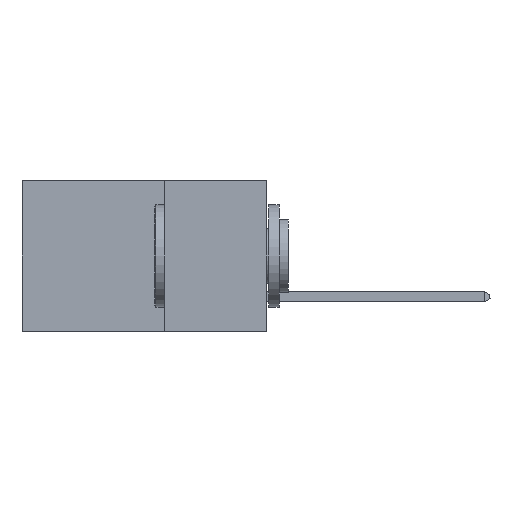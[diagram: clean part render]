
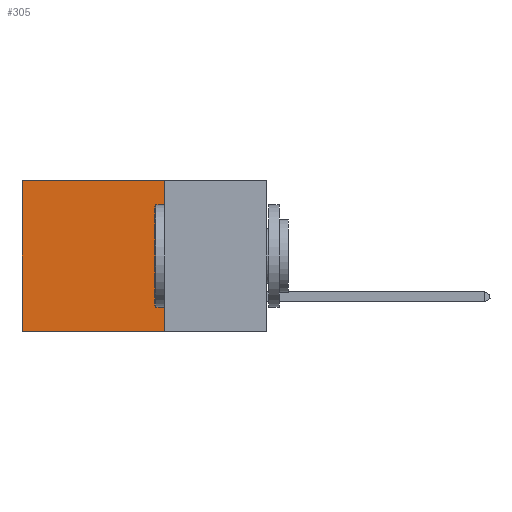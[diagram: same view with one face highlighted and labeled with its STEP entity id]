
A CAD part, left-side view. The second image highlights one B-rep face of the part: STEP entity #305.
In plain terms, the highlighted planar face has unit normal (-1, 0, 0).
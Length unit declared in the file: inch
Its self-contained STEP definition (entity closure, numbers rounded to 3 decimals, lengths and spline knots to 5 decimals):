
#305 = ADVANCED_FACE ( 'NONE', ( #17770 ), #11536, .F. ) ;
#1922 = ORIENTED_EDGE ( 'NONE', *, *, #16157, .F. ) ;
#2717 = EDGE_LOOP ( 'NONE', ( #24050, #1922, #35778, #18576 ) ) ;
#6690 = VERTEX_POINT ( 'NONE', #21975 ) ;
#7253 = LINE ( 'NONE', #20893, #22119 ) ;
#8516 = CARTESIAN_POINT ( 'NONE',  ( 0.2875, 0.25, 0. ) ) ;
#11536 = PLANE ( 'NONE',  #38023 ) ;
#11896 = CARTESIAN_POINT ( 'NONE',  ( 0.2875, 0.25, 0. ) ) ;
#12850 = LINE ( 'NONE', #30334, #37197 ) ;
#16157 = EDGE_CURVE ( 'NONE', #17183, #26474, #7253, .T. ) ;
#17183 = VERTEX_POINT ( 'NONE', #22636 ) ;
#17770 = FACE_OUTER_BOUND ( 'NONE', #2717, .T. ) ;
#18576 = ORIENTED_EDGE ( 'NONE', *, *, #26030, .T. ) ;
#19178 = LINE ( 'NONE', #8516, #35517 ) ;
#20381 = DIRECTION ( 'NONE',  ( 0., 0., -1. ) ) ;
#20893 = CARTESIAN_POINT ( 'NONE',  ( 0.2875, 0.25, -0.37 ) ) ;
#20948 = CARTESIAN_POINT ( 'NONE',  ( 0.2875, 0.25, 0. ) ) ;
#21975 = CARTESIAN_POINT ( 'NONE',  ( 0.2875, 0.6, 0. ) ) ;
#22119 = VECTOR ( 'NONE', #27307, 39.37008 ) ;
#22636 = CARTESIAN_POINT ( 'NONE',  ( 0.2875, 0.25, -0.37 ) ) ;
#23299 = CARTESIAN_POINT ( 'NONE',  ( 0.2875, 0.6, 0. ) ) ;
#23876 = DIRECTION ( 'NONE',  ( 1., 0., 0. ) ) ;
#24050 = ORIENTED_EDGE ( 'NONE', *, *, #34087, .T. ) ;
#26030 = EDGE_CURVE ( 'NONE', #40151, #6690, #12850, .T. ) ;
#26474 = VERTEX_POINT ( 'NONE', #40193 ) ;
#27307 = DIRECTION ( 'NONE',  ( 0., 1., 0. ) ) ;
#27555 = EDGE_CURVE ( 'NONE', #40151, #17183, #19178, .T. ) ;
#27655 = DIRECTION ( 'NONE',  ( 0., 0., -1. ) ) ;
#29329 = VECTOR ( 'NONE', #29681, 39.37008 ) ;
#29674 = DIRECTION ( 'NONE',  ( 0., 1., 0. ) ) ;
#29681 = DIRECTION ( 'NONE',  ( 0., 0., -1. ) ) ;
#30334 = CARTESIAN_POINT ( 'NONE',  ( 0.2875, 0.25, 0. ) ) ;
#34087 = EDGE_CURVE ( 'NONE', #6690, #26474, #37202, .T. ) ;
#35517 = VECTOR ( 'NONE', #27655, 39.37008 ) ;
#35778 = ORIENTED_EDGE ( 'NONE', *, *, #27555, .F. ) ;
#37197 = VECTOR ( 'NONE', #29674, 39.37008 ) ;
#37202 = LINE ( 'NONE', #23299, #29329 ) ;
#38023 = AXIS2_PLACEMENT_3D ( 'NONE', #20948, #23876, #20381 ) ;
#40151 = VERTEX_POINT ( 'NONE', #11896 ) ;
#40193 = CARTESIAN_POINT ( 'NONE',  ( 0.2875, 0.6, -0.37 ) ) ;
